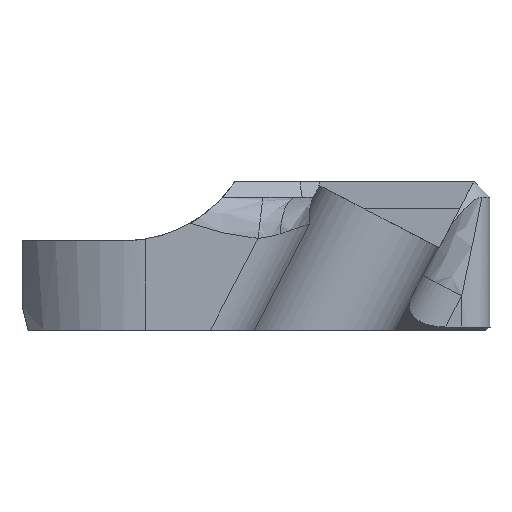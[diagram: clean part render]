
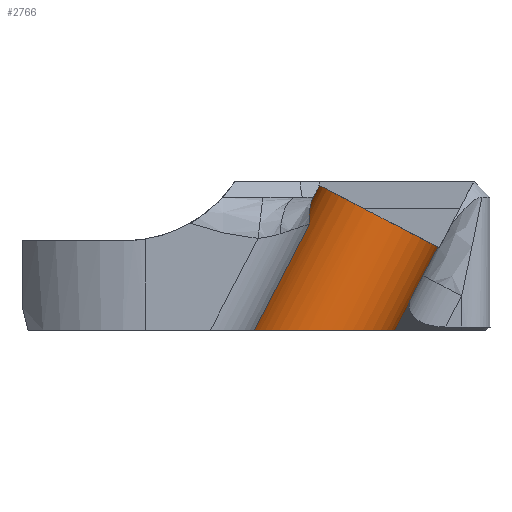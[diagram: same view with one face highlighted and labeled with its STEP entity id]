
A CAD part, front view. The second image highlights one B-rep face of the part: STEP entity #2766.
In plain terms, the highlighted cylindrical face has radius 9.525 mm (diameter 19.05 mm), a partial arc.
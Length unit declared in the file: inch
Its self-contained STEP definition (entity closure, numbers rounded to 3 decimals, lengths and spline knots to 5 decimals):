
#62 = B_SPLINE_CURVE_WITH_KNOTS ( 'NONE', 3,
 ( #5012, #9224, #5649, #4915, #749, #624, #6412, #1405, #2014, #5743, #5618, #4228 ),
 .UNSPECIFIED., .F., .F.,
 ( 4, 2, 2, 2, 2, 4 ),
 ( 0., 0.00288, 0.00432, 0.00504, 0.00541, 0.00577 ),
 .UNSPECIFIED. ) ;
#327 = CYLINDRICAL_SURFACE ( 'NONE', #4380, 0.375 ) ;
#345 = EDGE_LOOP ( 'NONE', ( #8422, #4851, #3745, #2905, #4647, #4043, #797, #6173, #1122 ) ) ;
#360 = EDGE_CURVE ( 'NONE', #3037, #3254, #2294, .T. ) ;
#417 = CARTESIAN_POINT ( 'NONE',  ( 4.04743, -0.41031, 3.25964 ) ) ;
#449 = DIRECTION ( 'NONE',  ( 0.887, 0., -0.461 ) ) ;
#605 = DIRECTION ( 'NONE',  ( -0.461, 0., -0.887 ) ) ;
#624 = CARTESIAN_POINT ( 'NONE',  ( 3.56557, -0.56042, 3.89086 ) ) ;
#716 = VECTOR ( 'NONE', #605, 39.37008 ) ;
#729 = VECTOR ( 'NONE', #4386, 39.37008 ) ;
#749 = CARTESIAN_POINT ( 'NONE',  ( 3.566, -0.53943, 3.91048 ) ) ;
#797 = ORIENTED_EDGE ( 'NONE', *, *, #4297, .F. ) ;
#803 = CARTESIAN_POINT ( 'NONE',  ( 3.62432, -0.41031, 4.07162 ) ) ;
#815 =( BOUNDED_CURVE ( )  B_SPLINE_CURVE ( 3, ( #8482, #1402, #4943, #8576 ),
 .UNSPECIFIED., .F., .T. ) 
 B_SPLINE_CURVE_WITH_KNOTS ( ( 4, 4 ),
 ( 0., 2.63168 ),
 .UNSPECIFIED. ) 
 CURVE ( )  GEOMETRIC_REPRESENTATION_ITEM ( )  RATIONAL_B_SPLINE_CURVE ( ( 1., 0.501, 0.501, 1. ) ) 
 REPRESENTATION_ITEM ( '' )  );
#1030 = CARTESIAN_POINT ( 'NONE',  ( 4.12321, -0.42711, 3.40537 ) ) ;
#1122 = ORIENTED_EDGE ( 'NONE', *, *, #5943, .T. ) ;
#1240 = CARTESIAN_POINT ( 'NONE',  ( 3.95702, -0.41031, 3.89861 ) ) ;
#1402 = CARTESIAN_POINT ( 'NONE',  ( 4.04743, -0.89273, 3.25964 ) ) ;
#1405 = CARTESIAN_POINT ( 'NONE',  ( 3.56561, -0.57722, 3.87381 ) ) ;
#1416 = CARTESIAN_POINT ( 'NONE',  ( 3.43597, -0.59335, 3.606 ) ) ;
#1720 = EDGE_CURVE ( 'NONE', #7239, #5209, #5416, .T. ) ;
#1879 = DIRECTION ( 'NONE',  ( 0.461, 0., 0.887 ) ) ;
#2014 = CARTESIAN_POINT ( 'NONE',  ( 3.56566, -0.5805, 3.87033 ) ) ;
#2246 = DIRECTION ( 'NONE',  ( 0.461, 0., 0.887 ) ) ;
#2294 = LINE ( 'NONE', #8617, #3963 ) ;
#2315 = CARTESIAN_POINT ( 'NONE',  ( 4.20316, -0.46052, 3.56645 ) ) ;
#2366 = VERTEX_POINT ( 'NONE', #417 ) ;
#2720 = LINE ( 'NONE', #8707, #729 ) ;
#2762 = CARTESIAN_POINT ( 'NONE',  ( 3.58083, -0.41031, 3.98799 ) ) ;
#2766 = ADVANCED_FACE ( 'NONE', ( #6950 ), #327, .T. ) ;
#2905 = ORIENTED_EDGE ( 'NONE', *, *, #360, .F. ) ;
#3005 = CARTESIAN_POINT ( 'NONE',  ( 4.11709, -0.41031, 3.39361 ) ) ;
#3037 = VERTEX_POINT ( 'NONE', #2762 ) ;
#3254 = VERTEX_POINT ( 'NONE', #803 ) ;
#3546 = DIRECTION ( 'NONE',  ( 0.461, 0., 0.887 ) ) ;
#3549 = DIRECTION ( 'NONE',  ( 0.887, 0., -0.461 ) ) ;
#3745 = ORIENTED_EDGE ( 'NONE', *, *, #8281, .F. ) ;
#3830 = CARTESIAN_POINT ( 'NONE',  ( 4.23104, -0.46052, 3.62007 ) ) ;
#3963 = VECTOR ( 'NONE', #3546, 39.37008 ) ;
#4043 = ORIENTED_EDGE ( 'NONE', *, *, #5058, .T. ) ;
#4165 = VECTOR ( 'NONE', #8887, 39.37008 ) ;
#4228 = CARTESIAN_POINT ( 'NONE',  ( 3.56604, -0.59335, 3.85614 ) ) ;
#4297 = EDGE_CURVE ( 'NONE', #2366, #4595, #815, .T. ) ;
#4380 = AXIS2_PLACEMENT_3D ( 'NONE', #6557, #2246, #3549 ) ;
#4386 = DIRECTION ( 'NONE',  ( 0.461, 0., 0.887 ) ) ;
#4500 = VERTEX_POINT ( 'NONE', #6478 ) ;
#4560 = EDGE_CURVE ( 'NONE', #4500, #7239, #2720, .T. ) ;
#4581 = CARTESIAN_POINT ( 'NONE',  ( 4.11709, -0.41031, 3.39361 ) ) ;
#4595 = VERTEX_POINT ( 'NONE', #8606 ) ;
#4647 = ORIENTED_EDGE ( 'NONE', *, *, #5794, .T. ) ;
#4851 = ORIENTED_EDGE ( 'NONE', *, *, #1720, .T. ) ;
#4915 = CARTESIAN_POINT ( 'NONE',  ( 3.5667, -0.52471, 3.92283 ) ) ;
#4943 = CARTESIAN_POINT ( 'NONE',  ( 3.52126, -1.0144, 3.25964 ) ) ;
#5012 = CARTESIAN_POINT ( 'NONE',  ( 3.58083, -0.41031, 3.98799 ) ) ;
#5022 = CARTESIAN_POINT ( 'NONE',  ( 3.56604, -0.59335, 3.85614 ) ) ;
#5058 = EDGE_CURVE ( 'NONE', #8608, #4595, #5747, .T. ) ;
#5116 = CARTESIAN_POINT ( 'NONE',  ( 4.28734, -0.45521, 3.72685 ) ) ;
#5209 = VERTEX_POINT ( 'NONE', #5116 ) ;
#5416 = B_SPLINE_CURVE_WITH_KNOTS ( 'NONE', 3,
 ( #2315, #3830, #6720, #7305 ),
 .UNSPECIFIED., .F., .F.,
 ( 4, 4 ),
 ( 0., 0.0046 ),
 .UNSPECIFIED. ) ;
#5428 = CIRCLE ( 'NONE', #8041, 0.375 ) ;
#5618 = CARTESIAN_POINT ( 'NONE',  ( 3.56591, -0.59023, 3.85969 ) ) ;
#5649 = CARTESIAN_POINT ( 'NONE',  ( 3.57015, -0.47876, 3.95677 ) ) ;
#5743 = CARTESIAN_POINT ( 'NONE',  ( 3.56581, -0.58699, 3.86329 ) ) ;
#5747 = LINE ( 'NONE', #1416, #716 ) ;
#5794 = EDGE_CURVE ( 'NONE', #3037, #8608, #62, .T. ) ;
#5926 = EDGE_CURVE ( 'NONE', #2366, #7995, #8336, .T. ) ;
#5943 = EDGE_CURVE ( 'NONE', #7995, #4500, #6502, .T. ) ;
#6066 = CARTESIAN_POINT ( 'NONE',  ( 4.12804, -0.44387, 3.41711 ) ) ;
#6173 = ORIENTED_EDGE ( 'NONE', *, *, #5926, .T. ) ;
#6412 = CARTESIAN_POINT ( 'NONE',  ( 3.56553, -0.56724, 3.88413 ) ) ;
#6478 = CARTESIAN_POINT ( 'NONE',  ( 4.13157, -0.46052, 3.42876 ) ) ;
#6502 =( BOUNDED_CURVE ( )  B_SPLINE_CURVE ( 3, ( #4581, #1030, #6066, #6798 ),
 .UNSPECIFIED., .F., .T. ) 
 B_SPLINE_CURVE_WITH_KNOTS ( ( 4, 4 ),
 ( 5.29498, 5.42926 ),
 .UNSPECIFIED. ) 
 CURVE ( )  GEOMETRIC_REPRESENTATION_ITEM ( )  RATIONAL_B_SPLINE_CURVE ( ( 1., 0.998, 0.998, 1. ) ) 
 REPRESENTATION_ITEM ( '' )  );
#6557 = CARTESIAN_POINT ( 'NONE',  ( 3.72635, -0.41031, 3.45501 ) ) ;
#6720 = CARTESIAN_POINT ( 'NONE',  ( 4.25912, -0.45882, 3.67353 ) ) ;
#6798 = CARTESIAN_POINT ( 'NONE',  ( 4.13157, -0.46052, 3.42876 ) ) ;
#6950 = FACE_OUTER_BOUND ( 'NONE', #345, .T. ) ;
#7239 = VERTEX_POINT ( 'NONE', #9169 ) ;
#7305 = CARTESIAN_POINT ( 'NONE',  ( 4.28734, -0.45521, 3.72685 ) ) ;
#7427 = CARTESIAN_POINT ( 'NONE',  ( 4.05905, -0.41031, 3.282 ) ) ;
#7995 = VERTEX_POINT ( 'NONE', #3005 ) ;
#8041 = AXIS2_PLACEMENT_3D ( 'NONE', #1240, #1879, #449 ) ;
#8281 = EDGE_CURVE ( 'NONE', #3254, #5209, #5428, .T. ) ;
#8336 = LINE ( 'NONE', #7427, #4165 ) ;
#8422 = ORIENTED_EDGE ( 'NONE', *, *, #4560, .T. ) ;
#8482 = CARTESIAN_POINT ( 'NONE',  ( 4.04743, -0.41031, 3.25964 ) ) ;
#8576 = CARTESIAN_POINT ( 'NONE',  ( 3.25586, -0.59335, 3.25964 ) ) ;
#8606 = CARTESIAN_POINT ( 'NONE',  ( 3.25586, -0.59335, 3.25964 ) ) ;
#8608 = VERTEX_POINT ( 'NONE', #5022 ) ;
#8617 = CARTESIAN_POINT ( 'NONE',  ( 3.39364, -0.41031, 3.62801 ) ) ;
#8707 = CARTESIAN_POINT ( 'NONE',  ( 4.05606, -0.46052, 3.28356 ) ) ;
#8887 = DIRECTION ( 'NONE',  ( 0.461, 0., 0.887 ) ) ;
#9169 = CARTESIAN_POINT ( 'NONE',  ( 4.20316, -0.46052, 3.56645 ) ) ;
#9224 = CARTESIAN_POINT ( 'NONE',  ( 3.57419, -0.44598, 3.97523 ) ) ;
